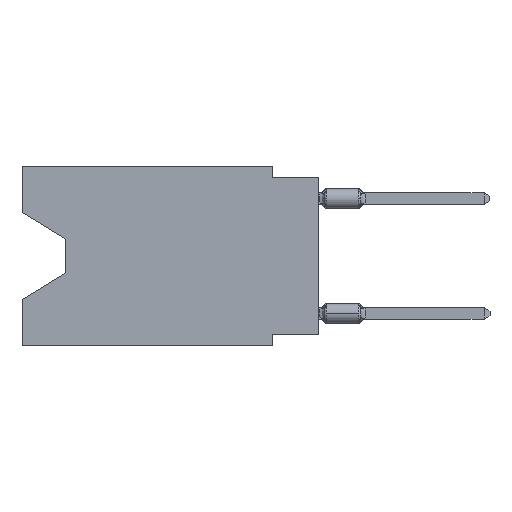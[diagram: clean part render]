
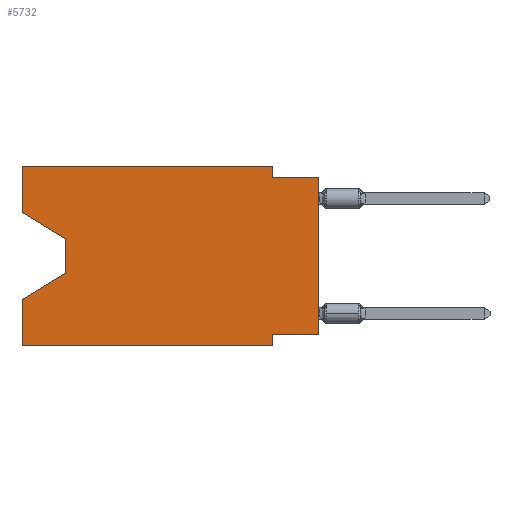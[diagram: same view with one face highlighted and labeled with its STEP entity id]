
A CAD part, left-side view. The second image highlights one B-rep face of the part: STEP entity #5732.
In plain terms, the highlighted planar face has unit normal (-1, 0, 0).
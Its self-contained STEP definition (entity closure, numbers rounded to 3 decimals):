
#2 = LINE ( 'NONE', #15188, #2637 ) ;
#328 = DIRECTION ( 'NONE',  ( 0., 0., -1. ) ) ;
#398 = CARTESIAN_POINT ( 'NONE',  ( 0., 2.54, -0.635 ) ) ;
#1052 = DIRECTION ( 'NONE',  ( 0., 0.855, -0.519 ) ) ;
#1172 = LINE ( 'NONE', #8892, #9911 ) ;
#1405 = CARTESIAN_POINT ( 'NONE',  ( 0., 2.54, -9.271 ) ) ;
#1541 = EDGE_CURVE ( 'NONE', #3271, #3516, #7570, .T. ) ;
#1616 = DIRECTION ( 'NONE',  ( 0., 1., 0. ) ) ;
#1948 = DIRECTION ( 'NONE',  ( 0., 0., 1. ) ) ;
#2079 = ORIENTED_EDGE ( 'NONE', *, *, #14540, .F. ) ;
#2637 = VECTOR ( 'NONE', #20704, 1000. ) ;
#2661 = CARTESIAN_POINT ( 'NONE',  ( 0., 13.97, -5.893 ) ) ;
#2814 = DIRECTION ( 'NONE',  ( 1., 0., 0. ) ) ;
#3237 = EDGE_CURVE ( 'NONE', #20310, #10081, #1172, .T. ) ;
#3257 = ORIENTED_EDGE ( 'NONE', *, *, #13470, .F. ) ;
#3271 = VERTEX_POINT ( 'NONE', #23564 ) ;
#3452 = EDGE_CURVE ( 'NONE', #19935, #10141, #5805, .T. ) ;
#3516 = VERTEX_POINT ( 'NONE', #17668 ) ;
#3642 = LINE ( 'NONE', #22359, #17746 ) ;
#3852 = CARTESIAN_POINT ( 'NONE',  ( 0., 0., -0.635 ) ) ;
#3922 = ORIENTED_EDGE ( 'NONE', *, *, #1541, .F. ) ;
#4011 = VERTEX_POINT ( 'NONE', #398 ) ;
#4106 = ORIENTED_EDGE ( 'NONE', *, *, #3237, .F. ) ;
#4135 = AXIS2_PLACEMENT_3D ( 'NONE', #8570, #2814, #17750 ) ;
#4838 = VERTEX_POINT ( 'NONE', #1405 ) ;
#5732 = ADVANCED_FACE ( 'NONE', ( #12130 ), #19588, .F. ) ;
#5788 = EDGE_CURVE ( 'NONE', #22009, #8786, #12859, .T. ) ;
#5805 = LINE ( 'NONE', #14981, #15377 ) ;
#6040 = CARTESIAN_POINT ( 'NONE',  ( 0., 16.383, 0. ) ) ;
#6210 = EDGE_CURVE ( 'NONE', #15157, #19935, #22353, .T. ) ;
#6539 = CARTESIAN_POINT ( 'NONE',  ( 0., 16.383, -7.36 ) ) ;
#6995 = CARTESIAN_POINT ( 'NONE',  ( 0., 16.383, -9.906 ) ) ;
#7402 = DIRECTION ( 'NONE',  ( 0., 0., -1. ) ) ;
#7570 = LINE ( 'NONE', #14807, #16097 ) ;
#7918 = VERTEX_POINT ( 'NONE', #18427 ) ;
#8399 = ORIENTED_EDGE ( 'NONE', *, *, #19035, .F. ) ;
#8570 = CARTESIAN_POINT ( 'NONE',  ( 0., 16.383, 0. ) ) ;
#8786 = VERTEX_POINT ( 'NONE', #3852 ) ;
#8892 = CARTESIAN_POINT ( 'NONE',  ( 0., 16.383, 0. ) ) ;
#9059 = LINE ( 'NONE', #9182, #21752 ) ;
#9182 = CARTESIAN_POINT ( 'NONE',  ( 0., 0., -0.635 ) ) ;
#9206 = CARTESIAN_POINT ( 'NONE',  ( 0., 0., -9.271 ) ) ;
#9738 = EDGE_CURVE ( 'NONE', #10141, #10081, #17947, .T. ) ;
#9911 = VECTOR ( 'NONE', #19913, 1000. ) ;
#10081 = VERTEX_POINT ( 'NONE', #6539 ) ;
#10141 = VERTEX_POINT ( 'NONE', #21709 ) ;
#10577 = EDGE_CURVE ( 'NONE', #4011, #8786, #9059, .T. ) ;
#11006 = EDGE_LOOP ( 'NONE', ( #20264, #12391, #21527, #4106, #12047, #13339, #3257, #13341, #13649, #8399, #3922, #2079 ) ) ;
#11143 = CARTESIAN_POINT ( 'NONE',  ( 0., 0., 0. ) ) ;
#11876 = EDGE_CURVE ( 'NONE', #4838, #7918, #2, .T. ) ;
#12047 = ORIENTED_EDGE ( 'NONE', *, *, #13731, .T. ) ;
#12130 = FACE_OUTER_BOUND ( 'NONE', #11006, .T. ) ;
#12136 = DIRECTION ( 'NONE',  ( 0., -1., 0. ) ) ;
#12364 = CARTESIAN_POINT ( 'NONE',  ( 0., 0., -9.271 ) ) ;
#12391 = ORIENTED_EDGE ( 'NONE', *, *, #3452, .T. ) ;
#12859 = LINE ( 'NONE', #11143, #20547 ) ;
#13339 = ORIENTED_EDGE ( 'NONE', *, *, #11876, .F. ) ;
#13341 = ORIENTED_EDGE ( 'NONE', *, *, #5788, .T. ) ;
#13470 = EDGE_CURVE ( 'NONE', #22009, #4838, #20355, .T. ) ;
#13521 = DIRECTION ( 'NONE',  ( 0., 0., 1. ) ) ;
#13649 = ORIENTED_EDGE ( 'NONE', *, *, #10577, .F. ) ;
#13731 = EDGE_CURVE ( 'NONE', #20310, #7918, #17760, .T. ) ;
#14540 = EDGE_CURVE ( 'NONE', #15157, #3271, #15346, .T. ) ;
#14651 = CARTESIAN_POINT ( 'NONE',  ( 0., 16.383, -2.546 ) ) ;
#14807 = CARTESIAN_POINT ( 'NONE',  ( 0., 16.383, 0. ) ) ;
#14981 = CARTESIAN_POINT ( 'NONE',  ( 0., 13.97, -4.013 ) ) ;
#15053 = VECTOR ( 'NONE', #13521, 1000. ) ;
#15157 = VERTEX_POINT ( 'NONE', #22395 ) ;
#15188 = CARTESIAN_POINT ( 'NONE',  ( 0., 2.54, -9.906 ) ) ;
#15346 = LINE ( 'NONE', #6040, #15053 ) ;
#15377 = VECTOR ( 'NONE', #7402, 1000. ) ;
#16097 = VECTOR ( 'NONE', #20688, 1000. ) ;
#16354 = VECTOR ( 'NONE', #1616, 1000. ) ;
#17668 = CARTESIAN_POINT ( 'NONE',  ( 0., 2.54, 0. ) ) ;
#17746 = VECTOR ( 'NONE', #328, 1000. ) ;
#17750 = DIRECTION ( 'NONE',  ( 0., 0., -1. ) ) ;
#17760 = LINE ( 'NONE', #21805, #20516 ) ;
#17947 = LINE ( 'NONE', #2661, #18587 ) ;
#18427 = CARTESIAN_POINT ( 'NONE',  ( 0., 2.54, -9.906 ) ) ;
#18587 = VECTOR ( 'NONE', #1052, 1000. ) ;
#19035 = EDGE_CURVE ( 'NONE', #3516, #4011, #3642, .T. ) ;
#19588 = PLANE ( 'NONE',  #4135 ) ;
#19856 = DIRECTION ( 'NONE',  ( 0., -1., 0. ) ) ;
#19913 = DIRECTION ( 'NONE',  ( 0., 0., 1. ) ) ;
#19935 = VERTEX_POINT ( 'NONE', #22779 ) ;
#20264 = ORIENTED_EDGE ( 'NONE', *, *, #6210, .T. ) ;
#20310 = VERTEX_POINT ( 'NONE', #6995 ) ;
#20355 = LINE ( 'NONE', #9206, #16354 ) ;
#20516 = VECTOR ( 'NONE', #12136, 1000. ) ;
#20547 = VECTOR ( 'NONE', #1948, 1000. ) ;
#20688 = DIRECTION ( 'NONE',  ( 0., -1., 0. ) ) ;
#20704 = DIRECTION ( 'NONE',  ( 0., 0., -1. ) ) ;
#21527 = ORIENTED_EDGE ( 'NONE', *, *, #9738, .T. ) ;
#21709 = CARTESIAN_POINT ( 'NONE',  ( 0., 13.97, -5.893 ) ) ;
#21752 = VECTOR ( 'NONE', #19856, 1000. ) ;
#21753 = VECTOR ( 'NONE', #23943, 1000. ) ;
#21805 = CARTESIAN_POINT ( 'NONE',  ( 0., 16.383, -9.906 ) ) ;
#22009 = VERTEX_POINT ( 'NONE', #12364 ) ;
#22353 = LINE ( 'NONE', #14651, #21753 ) ;
#22359 = CARTESIAN_POINT ( 'NONE',  ( 0., 2.54, 0. ) ) ;
#22395 = CARTESIAN_POINT ( 'NONE',  ( 0., 16.383, -2.546 ) ) ;
#22779 = CARTESIAN_POINT ( 'NONE',  ( 0., 13.97, -4.013 ) ) ;
#23564 = CARTESIAN_POINT ( 'NONE',  ( 0., 16.383, 0. ) ) ;
#23943 = DIRECTION ( 'NONE',  ( 0., -0.855, -0.519 ) ) ;
